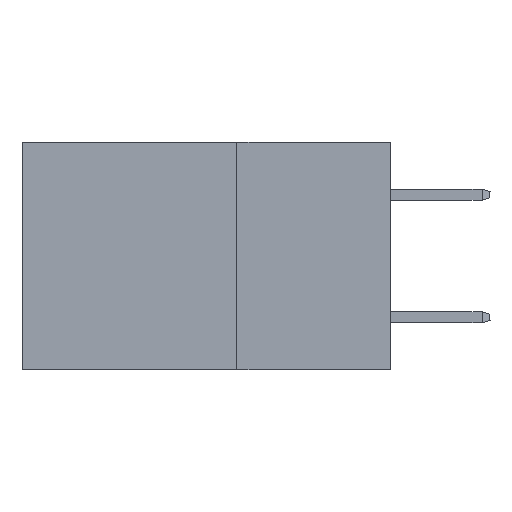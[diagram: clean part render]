
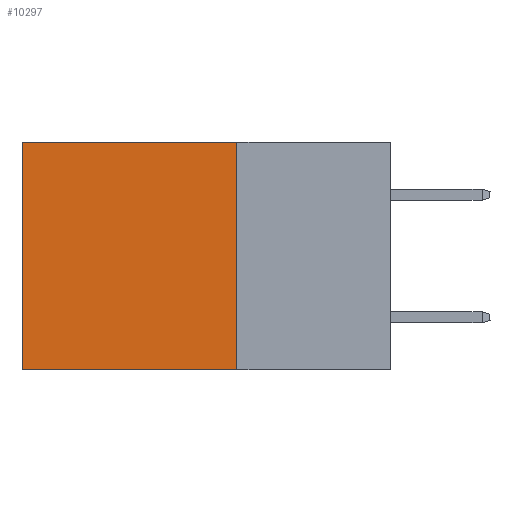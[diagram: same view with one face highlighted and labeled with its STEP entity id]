
A CAD part, left-side view. The second image highlights one B-rep face of the part: STEP entity #10297.
In plain terms, the highlighted planar face has unit normal (-1, 0, 0).
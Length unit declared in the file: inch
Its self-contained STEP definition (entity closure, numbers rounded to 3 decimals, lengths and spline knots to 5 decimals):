
#68 = DIRECTION ( 'NONE',  ( 0., 0., -1. ) ) ;
#86 = LINE ( 'NONE', #15541, #6808 ) ;
#371 = DIRECTION ( 'NONE',  ( 1., 0., 0. ) ) ;
#485 = ORIENTED_EDGE ( 'NONE', *, *, #12099, .F. ) ;
#626 = CARTESIAN_POINT ( 'NONE',  ( 0.2875, 0.25, -0.37 ) ) ;
#1777 = LINE ( 'NONE', #14029, #14629 ) ;
#2786 = VERTEX_POINT ( 'NONE', #6231 ) ;
#3103 = DIRECTION ( 'NONE',  ( 0., 0., -1. ) ) ;
#4301 = CARTESIAN_POINT ( 'NONE',  ( 0.2875, 0.6, 0. ) ) ;
#4861 = EDGE_CURVE ( 'NONE', #11498, #5601, #1777, .T. ) ;
#4971 = AXIS2_PLACEMENT_3D ( 'NONE', #10814, #371, #9591 ) ;
#5103 = CARTESIAN_POINT ( 'NONE',  ( 0.2875, 0.25, -0.37 ) ) ;
#5455 = ORIENTED_EDGE ( 'NONE', *, *, #4861, .T. ) ;
#5566 = FACE_OUTER_BOUND ( 'NONE', #14580, .T. ) ;
#5601 = VERTEX_POINT ( 'NONE', #4301 ) ;
#6231 = CARTESIAN_POINT ( 'NONE',  ( 0.2875, 0.6, -0.37 ) ) ;
#6307 = VECTOR ( 'NONE', #3103, 39.37008 ) ;
#6808 = VECTOR ( 'NONE', #68, 39.37008 ) ;
#7764 = DIRECTION ( 'NONE',  ( 0., 1., 0. ) ) ;
#9591 = DIRECTION ( 'NONE',  ( 0., 0., -1. ) ) ;
#10000 = VERTEX_POINT ( 'NONE', #5103 ) ;
#10174 = EDGE_CURVE ( 'NONE', #5601, #2786, #86, .T. ) ;
#10297 = ADVANCED_FACE ( 'NONE', ( #5566 ), #15815, .F. ) ;
#10814 = CARTESIAN_POINT ( 'NONE',  ( 0.2875, 0.25, 0. ) ) ;
#10848 = CARTESIAN_POINT ( 'NONE',  ( 0.2875, 0.25, 0. ) ) ;
#11498 = VERTEX_POINT ( 'NONE', #15607 ) ;
#12099 = EDGE_CURVE ( 'NONE', #10000, #2786, #14406, .T. ) ;
#12340 = DIRECTION ( 'NONE',  ( 0., 1., 0. ) ) ;
#13037 = LINE ( 'NONE', #10848, #6307 ) ;
#13149 = EDGE_CURVE ( 'NONE', #11498, #10000, #13037, .T. ) ;
#14027 = VECTOR ( 'NONE', #12340, 39.37008 ) ;
#14029 = CARTESIAN_POINT ( 'NONE',  ( 0.2875, 0.25, 0. ) ) ;
#14406 = LINE ( 'NONE', #626, #14027 ) ;
#14580 = EDGE_LOOP ( 'NONE', ( #15068, #485, #16250, #5455 ) ) ;
#14629 = VECTOR ( 'NONE', #7764, 39.37008 ) ;
#15068 = ORIENTED_EDGE ( 'NONE', *, *, #10174, .T. ) ;
#15541 = CARTESIAN_POINT ( 'NONE',  ( 0.2875, 0.6, 0. ) ) ;
#15607 = CARTESIAN_POINT ( 'NONE',  ( 0.2875, 0.25, 0. ) ) ;
#15815 = PLANE ( 'NONE',  #4971 ) ;
#16250 = ORIENTED_EDGE ( 'NONE', *, *, #13149, .F. ) ;
